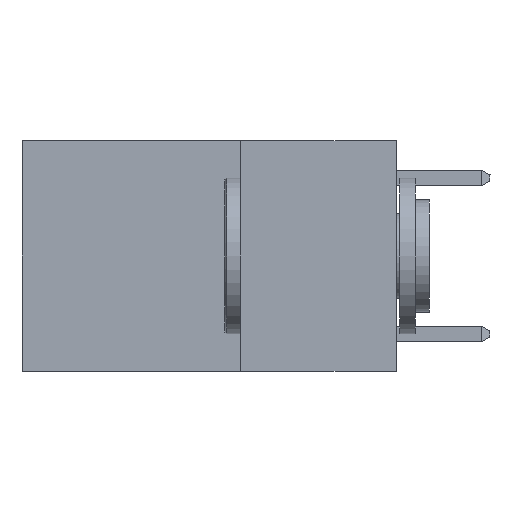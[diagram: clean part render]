
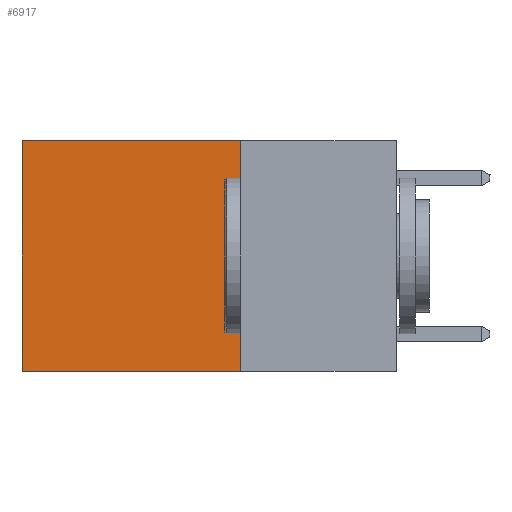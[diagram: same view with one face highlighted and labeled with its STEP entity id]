
A CAD part, left-side view. The second image highlights one B-rep face of the part: STEP entity #6917.
In plain terms, the highlighted planar face has unit normal (-1, 0, 0).
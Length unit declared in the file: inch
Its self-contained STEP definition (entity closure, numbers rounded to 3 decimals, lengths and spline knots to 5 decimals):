
#325 = CARTESIAN_POINT ( 'NONE',  ( 0.2625, 0.25, -0.37 ) ) ;
#397 = ORIENTED_EDGE ( 'NONE', *, *, #9361, .F. ) ;
#521 = CARTESIAN_POINT ( 'NONE',  ( 0.2625, 0.25, 0. ) ) ;
#522 = VERTEX_POINT ( 'NONE', #4016 ) ;
#656 = EDGE_CURVE ( 'NONE', #3560, #4155, #2175, .T. ) ;
#1608 = ORIENTED_EDGE ( 'NONE', *, *, #4874, .T. ) ;
#1868 = DIRECTION ( 'NONE',  ( 1., 0., 0. ) ) ;
#2175 = LINE ( 'NONE', #5256, #6008 ) ;
#2674 = VECTOR ( 'NONE', #4062, 39.37008 ) ;
#3394 = DIRECTION ( 'NONE',  ( 0., 0., -1. ) ) ;
#3560 = VERTEX_POINT ( 'NONE', #9215 ) ;
#4016 = CARTESIAN_POINT ( 'NONE',  ( 0.2625, 0.25, -0.37 ) ) ;
#4062 = DIRECTION ( 'NONE',  ( 0., 0., -1. ) ) ;
#4075 = ORIENTED_EDGE ( 'NONE', *, *, #4197, .F. ) ;
#4155 = VERTEX_POINT ( 'NONE', #8953 ) ;
#4197 = EDGE_CURVE ( 'NONE', #522, #6164, #4515, .T. ) ;
#4318 = CARTESIAN_POINT ( 'NONE',  ( 0.2625, 0.6, -0.37 ) ) ;
#4515 = LINE ( 'NONE', #325, #6656 ) ;
#4781 = LINE ( 'NONE', #7703, #2674 ) ;
#4874 = EDGE_CURVE ( 'NONE', #4155, #6164, #4781, .T. ) ;
#4881 = CARTESIAN_POINT ( 'NONE',  ( 0.2625, 0.25, 0. ) ) ;
#5256 = CARTESIAN_POINT ( 'NONE',  ( 0.2625, 0.25, 0. ) ) ;
#6008 = VECTOR ( 'NONE', #7395, 39.37008 ) ;
#6142 = DIRECTION ( 'NONE',  ( 0., 1., 0. ) ) ;
#6164 = VERTEX_POINT ( 'NONE', #4318 ) ;
#6171 = DIRECTION ( 'NONE',  ( 0., 0., -1. ) ) ;
#6656 = VECTOR ( 'NONE', #6142, 39.37008 ) ;
#6692 = AXIS2_PLACEMENT_3D ( 'NONE', #521, #1868, #6171 ) ;
#6917 = ADVANCED_FACE ( 'NONE', ( #7782 ), #9027, .F. ) ;
#7395 = DIRECTION ( 'NONE',  ( 0., 1., 0. ) ) ;
#7700 = LINE ( 'NONE', #4881, #8996 ) ;
#7703 = CARTESIAN_POINT ( 'NONE',  ( 0.2625, 0.6, 0. ) ) ;
#7782 = FACE_OUTER_BOUND ( 'NONE', #8609, .T. ) ;
#8029 = ORIENTED_EDGE ( 'NONE', *, *, #656, .T. ) ;
#8609 = EDGE_LOOP ( 'NONE', ( #1608, #4075, #397, #8029 ) ) ;
#8953 = CARTESIAN_POINT ( 'NONE',  ( 0.2625, 0.6, 0. ) ) ;
#8996 = VECTOR ( 'NONE', #3394, 39.37008 ) ;
#9027 = PLANE ( 'NONE',  #6692 ) ;
#9215 = CARTESIAN_POINT ( 'NONE',  ( 0.2625, 0.25, 0. ) ) ;
#9361 = EDGE_CURVE ( 'NONE', #3560, #522, #7700, .T. ) ;
